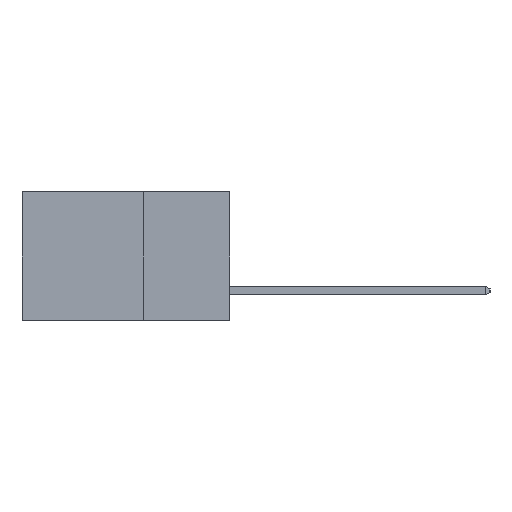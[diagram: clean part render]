
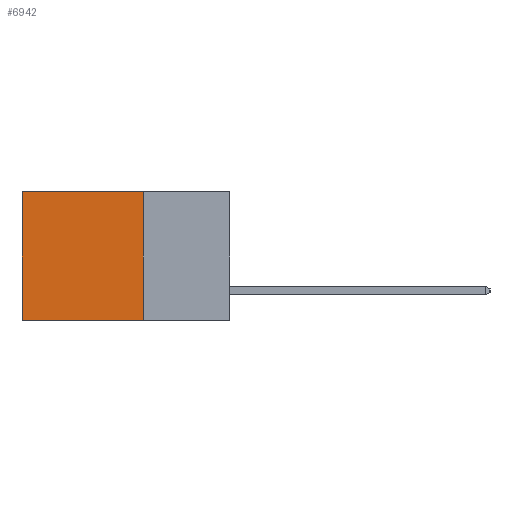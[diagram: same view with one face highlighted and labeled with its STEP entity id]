
A CAD part, left-side view. The second image highlights one B-rep face of the part: STEP entity #6942.
In plain terms, the highlighted planar face has unit normal (-1, 0, 0).
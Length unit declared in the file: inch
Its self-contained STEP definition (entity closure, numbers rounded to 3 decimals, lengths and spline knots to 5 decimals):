
#1172 = FACE_OUTER_BOUND ( 'NONE', #13290, .T. ) ;
#1391 = VERTEX_POINT ( 'NONE', #15081 ) ;
#2751 = VERTEX_POINT ( 'NONE', #17045 ) ;
#3239 = LINE ( 'NONE', #5490, #19861 ) ;
#5297 = EDGE_CURVE ( 'NONE', #19837, #2751, #10369, .T. ) ;
#5490 = CARTESIAN_POINT ( 'NONE',  ( 0.2615, 0.25, -0.37 ) ) ;
#5740 = VECTOR ( 'NONE', #8608, 39.37008 ) ;
#6210 = ORIENTED_EDGE ( 'NONE', *, *, #6501, .T. ) ;
#6501 = EDGE_CURVE ( 'NONE', #1391, #9596, #14519, .T. ) ;
#6942 = ADVANCED_FACE ( 'NONE', ( #1172 ), #12646, .F. ) ;
#7302 = VECTOR ( 'NONE', #19621, 39.37008 ) ;
#7701 = CARTESIAN_POINT ( 'NONE',  ( 0.2615, 0.25, 0. ) ) ;
#8608 = DIRECTION ( 'NONE',  ( 0., 0., -1. ) ) ;
#8684 = CARTESIAN_POINT ( 'NONE',  ( 0.2615, 0.25, -0.37 ) ) ;
#9596 = VERTEX_POINT ( 'NONE', #21435 ) ;
#10369 = LINE ( 'NONE', #8684, #5740 ) ;
#12030 = DIRECTION ( 'NONE',  ( 0., 0., -1. ) ) ;
#12048 = DIRECTION ( 'NONE',  ( 1., 0., 0. ) ) ;
#12126 = CARTESIAN_POINT ( 'NONE',  ( 0.2615, 0.25, -0.37 ) ) ;
#12646 = PLANE ( 'NONE',  #14335 ) ;
#12709 = ORIENTED_EDGE ( 'NONE', *, *, #17852, .F. ) ;
#12736 = EDGE_CURVE ( 'NONE', #19837, #1391, #20317, .T. ) ;
#13290 = EDGE_LOOP ( 'NONE', ( #6210, #12709, #15828, #19636 ) ) ;
#14335 = AXIS2_PLACEMENT_3D ( 'NONE', #12126, #12048, #12030 ) ;
#14519 = LINE ( 'NONE', #20728, #18946 ) ;
#15081 = CARTESIAN_POINT ( 'NONE',  ( 0.2615, 0.6, 0. ) ) ;
#15828 = ORIENTED_EDGE ( 'NONE', *, *, #5297, .F. ) ;
#17045 = CARTESIAN_POINT ( 'NONE',  ( 0.2615, 0.25, -0.37 ) ) ;
#17852 = EDGE_CURVE ( 'NONE', #2751, #9596, #3239, .T. ) ;
#18583 = CARTESIAN_POINT ( 'NONE',  ( 0.2615, 0.25, 0. ) ) ;
#18946 = VECTOR ( 'NONE', #20767, 39.37008 ) ;
#19621 = DIRECTION ( 'NONE',  ( 0., 1., 0. ) ) ;
#19636 = ORIENTED_EDGE ( 'NONE', *, *, #12736, .T. ) ;
#19837 = VERTEX_POINT ( 'NONE', #18583 ) ;
#19861 = VECTOR ( 'NONE', #20791, 39.37008 ) ;
#20317 = LINE ( 'NONE', #7701, #7302 ) ;
#20728 = CARTESIAN_POINT ( 'NONE',  ( 0.2615, 0.6, -0.37 ) ) ;
#20767 = DIRECTION ( 'NONE',  ( 0., 0., -1. ) ) ;
#20791 = DIRECTION ( 'NONE',  ( 0., 1., 0. ) ) ;
#21435 = CARTESIAN_POINT ( 'NONE',  ( 0.2615, 0.6, -0.37 ) ) ;
